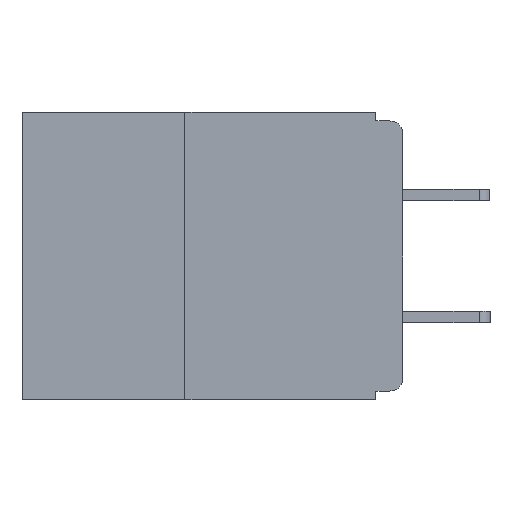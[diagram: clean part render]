
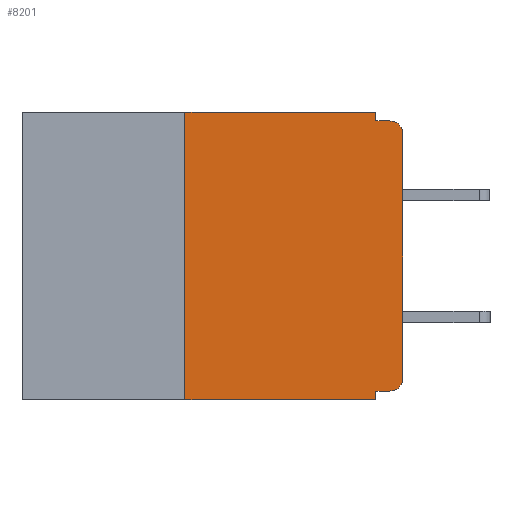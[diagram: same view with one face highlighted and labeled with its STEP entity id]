
A CAD part, left-side view. The second image highlights one B-rep face of the part: STEP entity #8201.
In plain terms, the highlighted planar face has unit normal (-1, 0, 0).
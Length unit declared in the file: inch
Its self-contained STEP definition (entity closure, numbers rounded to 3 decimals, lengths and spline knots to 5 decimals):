
#118 = CIRCLE ( 'NONE', #21468, 0.015 ) ;
#637 = LINE ( 'NONE', #5421, #15868 ) ;
#783 = DIRECTION ( 'NONE',  ( -1., 0., 0. ) ) ;
#851 = EDGE_CURVE ( 'NONE', #18130, #16450, #22620, .T. ) ;
#1148 = VECTOR ( 'NONE', #24098, 39.37008 ) ;
#1264 = CARTESIAN_POINT ( 'NONE',  ( 0., 0.015, -0.305 ) ) ;
#1475 = VERTEX_POINT ( 'NONE', #17031 ) ;
#2209 = ORIENTED_EDGE ( 'NONE', *, *, #14680, .T. ) ;
#2334 = VERTEX_POINT ( 'NONE', #7591 ) ;
#3265 = DIRECTION ( 'NONE',  ( 0., 0., -1. ) ) ;
#3616 = DIRECTION ( 'NONE',  ( 0., 0., -1. ) ) ;
#3673 = CARTESIAN_POINT ( 'NONE',  ( 0., 0.031, 0. ) ) ;
#3742 = DIRECTION ( 'NONE',  ( 0., 0., -1. ) ) ;
#3811 = CARTESIAN_POINT ( 'NONE',  ( 0., 0.031, -0.33 ) ) ;
#3872 = DIRECTION ( 'NONE',  ( 0., 0., -1. ) ) ;
#3904 = CARTESIAN_POINT ( 'NONE',  ( 0., 0.015, -0.025 ) ) ;
#4250 = VERTEX_POINT ( 'NONE', #15004 ) ;
#4405 = LINE ( 'NONE', #3811, #25190 ) ;
#4934 = EDGE_LOOP ( 'NONE', ( #23977, #9058, #6980, #20933, #12794, #13194, #19783, #20033, #10204, #2209 ) ) ;
#5373 = EDGE_CURVE ( 'NONE', #13561, #18122, #9452, .T. ) ;
#5421 = CARTESIAN_POINT ( 'NONE',  ( 0., 0., 0. ) ) ;
#5477 = VERTEX_POINT ( 'NONE', #19682 ) ;
#5605 = CARTESIAN_POINT ( 'NONE',  ( 0., 0., -0.025 ) ) ;
#5782 = EDGE_CURVE ( 'NONE', #18122, #14197, #5960, .T. ) ;
#5893 = DIRECTION ( 'NONE',  ( 0., 0., 1. ) ) ;
#5960 = LINE ( 'NONE', #3673, #15275 ) ;
#6171 = EDGE_CURVE ( 'NONE', #2334, #1475, #7546, .T. ) ;
#6572 = DIRECTION ( 'NONE',  ( 0., 0., -1. ) ) ;
#6596 = DIRECTION ( 'NONE',  ( 1., 0., 0. ) ) ;
#6686 = VECTOR ( 'NONE', #16574, 39.37008 ) ;
#6688 = CARTESIAN_POINT ( 'NONE',  ( 0., 0.437, 0. ) ) ;
#6722 = PLANE ( 'NONE',  #15855 ) ;
#6917 = VERTEX_POINT ( 'NONE', #22738 ) ;
#6980 = ORIENTED_EDGE ( 'NONE', *, *, #21550, .F. ) ;
#7546 = LINE ( 'NONE', #17740, #16818 ) ;
#7591 = CARTESIAN_POINT ( 'NONE',  ( 0., 0.015, -0.32 ) ) ;
#8201 = ADVANCED_FACE ( 'NONE', ( #10709 ), #6722, .F. ) ;
#8464 = EDGE_CURVE ( 'NONE', #1475, #5477, #4405, .T. ) ;
#9058 = ORIENTED_EDGE ( 'NONE', *, *, #851, .T. ) ;
#9078 = EDGE_CURVE ( 'NONE', #6917, #18130, #637, .T. ) ;
#9452 = LINE ( 'NONE', #24986, #24331 ) ;
#10204 = ORIENTED_EDGE ( 'NONE', *, *, #6171, .F. ) ;
#10709 = FACE_OUTER_BOUND ( 'NONE', #4934, .T. ) ;
#10806 = LINE ( 'NONE', #10859, #20602 ) ;
#10859 = CARTESIAN_POINT ( 'NONE',  ( 0., 0.437, -0.33 ) ) ;
#10987 = AXIS2_PLACEMENT_3D ( 'NONE', #3904, #783, #3872 ) ;
#12794 = ORIENTED_EDGE ( 'NONE', *, *, #5373, .F. ) ;
#13194 = ORIENTED_EDGE ( 'NONE', *, *, #22117, .F. ) ;
#13561 = VERTEX_POINT ( 'NONE', #23451 ) ;
#14197 = VERTEX_POINT ( 'NONE', #15418 ) ;
#14680 = EDGE_CURVE ( 'NONE', #2334, #6917, #118, .T. ) ;
#15004 = CARTESIAN_POINT ( 'NONE',  ( 0., 0.25, -0.33 ) ) ;
#15135 = DIRECTION ( 'NONE',  ( -1., 0., 0. ) ) ;
#15275 = VECTOR ( 'NONE', #3616, 39.37008 ) ;
#15418 = CARTESIAN_POINT ( 'NONE',  ( 0., 0.031, -0.01 ) ) ;
#15855 = AXIS2_PLACEMENT_3D ( 'NONE', #6688, #6596, #6572 ) ;
#15868 = VECTOR ( 'NONE', #5893, 39.37008 ) ;
#16450 = VERTEX_POINT ( 'NONE', #24720 ) ;
#16574 = DIRECTION ( 'NONE',  ( 0., 0., 1. ) ) ;
#16818 = VECTOR ( 'NONE', #17362, 39.37008 ) ;
#17031 = CARTESIAN_POINT ( 'NONE',  ( 0., 0.031, -0.32 ) ) ;
#17362 = DIRECTION ( 'NONE',  ( 0., 1., 0. ) ) ;
#17740 = CARTESIAN_POINT ( 'NONE',  ( 0., 0., -0.32 ) ) ;
#18122 = VERTEX_POINT ( 'NONE', #21308 ) ;
#18130 = VERTEX_POINT ( 'NONE', #5605 ) ;
#18652 = DIRECTION ( 'NONE',  ( 0., -1., 0. ) ) ;
#19682 = CARTESIAN_POINT ( 'NONE',  ( 0., 0.031, -0.33 ) ) ;
#19783 = ORIENTED_EDGE ( 'NONE', *, *, #20335, .T. ) ;
#20033 = ORIENTED_EDGE ( 'NONE', *, *, #8464, .F. ) ;
#20323 = LINE ( 'NONE', #24168, #1148 ) ;
#20335 = EDGE_CURVE ( 'NONE', #4250, #5477, #10806, .T. ) ;
#20602 = VECTOR ( 'NONE', #18652, 39.37008 ) ;
#20933 = ORIENTED_EDGE ( 'NONE', *, *, #5782, .F. ) ;
#21308 = CARTESIAN_POINT ( 'NONE',  ( 0., 0.031, 0. ) ) ;
#21468 = AXIS2_PLACEMENT_3D ( 'NONE', #1264, #15135, #3265 ) ;
#21550 = EDGE_CURVE ( 'NONE', #14197, #16450, #20323, .T. ) ;
#22117 = EDGE_CURVE ( 'NONE', #4250, #13561, #23550, .T. ) ;
#22441 = CARTESIAN_POINT ( 'NONE',  ( 0., 0.25, -0.33 ) ) ;
#22620 = CIRCLE ( 'NONE', #10987, 0.015 ) ;
#22738 = CARTESIAN_POINT ( 'NONE',  ( 0., 0., -0.305 ) ) ;
#23451 = CARTESIAN_POINT ( 'NONE',  ( 0., 0.25, 0. ) ) ;
#23550 = LINE ( 'NONE', #22441, #6686 ) ;
#23977 = ORIENTED_EDGE ( 'NONE', *, *, #9078, .T. ) ;
#24098 = DIRECTION ( 'NONE',  ( 0., -1., 0. ) ) ;
#24168 = CARTESIAN_POINT ( 'NONE',  ( 0., 0., -0.01 ) ) ;
#24331 = VECTOR ( 'NONE', #24364, 39.37008 ) ;
#24364 = DIRECTION ( 'NONE',  ( 0., -1., 0. ) ) ;
#24720 = CARTESIAN_POINT ( 'NONE',  ( 0., 0.015, -0.01 ) ) ;
#24986 = CARTESIAN_POINT ( 'NONE',  ( 0., 0.437, 0. ) ) ;
#25190 = VECTOR ( 'NONE', #3742, 39.37008 ) ;
